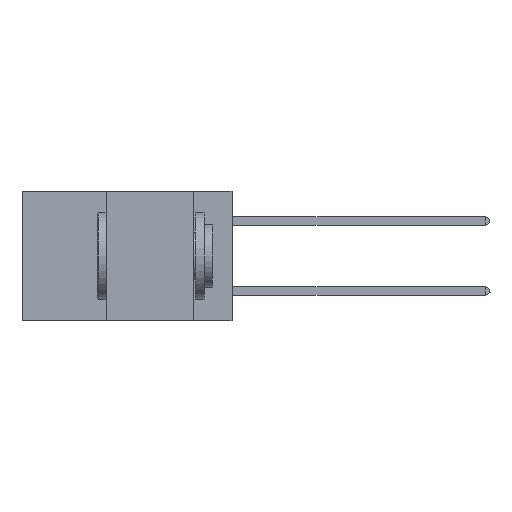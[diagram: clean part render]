
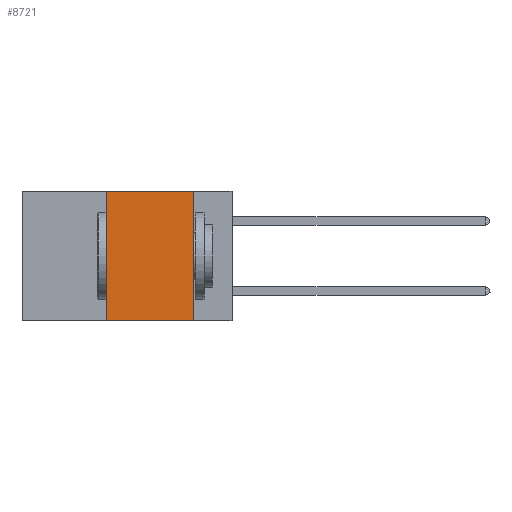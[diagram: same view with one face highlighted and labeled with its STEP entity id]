
A CAD part, left-side view. The second image highlights one B-rep face of the part: STEP entity #8721.
In plain terms, the highlighted planar face has unit normal (-1, 0, 0).
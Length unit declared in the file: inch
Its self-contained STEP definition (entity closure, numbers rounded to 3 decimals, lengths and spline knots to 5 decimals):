
#110 = VECTOR ( 'NONE', #27107, 39.37008 ) ;
#234 = EDGE_CURVE ( 'NONE', #19731, #16163, #21909, .T. ) ;
#271 = AXIS2_PLACEMENT_3D ( 'NONE', #6091, #6285, #10564 ) ;
#2709 = LINE ( 'NONE', #25144, #8342 ) ;
#3290 = EDGE_CURVE ( 'NONE', #8094, #19731, #2709, .T. ) ;
#3865 = PLANE ( 'NONE',  #271 ) ;
#6091 = CARTESIAN_POINT ( 'NONE',  ( 0., 0.6, 0. ) ) ;
#6285 = DIRECTION ( 'NONE',  ( 1., 0., 0. ) ) ;
#6864 = ORIENTED_EDGE ( 'NONE', *, *, #234, .F. ) ;
#8094 = VERTEX_POINT ( 'NONE', #14889 ) ;
#8152 = ORIENTED_EDGE ( 'NONE', *, *, #3290, .F. ) ;
#8342 = VECTOR ( 'NONE', #20914, 39.37008 ) ;
#8721 = ADVANCED_FACE ( 'NONE', ( #18894 ), #3865, .F. ) ;
#10564 = DIRECTION ( 'NONE',  ( 0., 0., -1. ) ) ;
#11238 = EDGE_CURVE ( 'NONE', #8094, #28241, #12965, .T. ) ;
#12222 = CARTESIAN_POINT ( 'NONE',  ( 0., 0.11, -0.37 ) ) ;
#12965 = LINE ( 'NONE', #25231, #17113 ) ;
#14889 = CARTESIAN_POINT ( 'NONE',  ( 0., 0.36, -0.37 ) ) ;
#14932 = EDGE_LOOP ( 'NONE', ( #24166, #6864, #8152, #27515 ) ) ;
#16163 = VERTEX_POINT ( 'NONE', #16247 ) ;
#16247 = CARTESIAN_POINT ( 'NONE',  ( 0., 0.11, 0. ) ) ;
#16955 = EDGE_CURVE ( 'NONE', #16163, #28241, #24035, .T. ) ;
#17113 = VECTOR ( 'NONE', #27435, 39.37008 ) ;
#17534 = DIRECTION ( 'NONE',  ( 0., 0., -1. ) ) ;
#18894 = FACE_OUTER_BOUND ( 'NONE', #14932, .T. ) ;
#19731 = VERTEX_POINT ( 'NONE', #27182 ) ;
#20914 = DIRECTION ( 'NONE',  ( 0., 0., 1. ) ) ;
#21909 = LINE ( 'NONE', #25006, #110 ) ;
#21946 = VECTOR ( 'NONE', #17534, 39.37008 ) ;
#23987 = CARTESIAN_POINT ( 'NONE',  ( 0., 0.11, 0. ) ) ;
#24035 = LINE ( 'NONE', #23987, #21946 ) ;
#24166 = ORIENTED_EDGE ( 'NONE', *, *, #16955, .F. ) ;
#25006 = CARTESIAN_POINT ( 'NONE',  ( 0., 0.6, 0. ) ) ;
#25144 = CARTESIAN_POINT ( 'NONE',  ( 0., 0.36, 0. ) ) ;
#25231 = CARTESIAN_POINT ( 'NONE',  ( 0., 0.6, -0.37 ) ) ;
#27107 = DIRECTION ( 'NONE',  ( 0., -1., 0. ) ) ;
#27182 = CARTESIAN_POINT ( 'NONE',  ( 0., 0.36, 0. ) ) ;
#27435 = DIRECTION ( 'NONE',  ( 0., -1., 0. ) ) ;
#27515 = ORIENTED_EDGE ( 'NONE', *, *, #11238, .T. ) ;
#28241 = VERTEX_POINT ( 'NONE', #12222 ) ;
